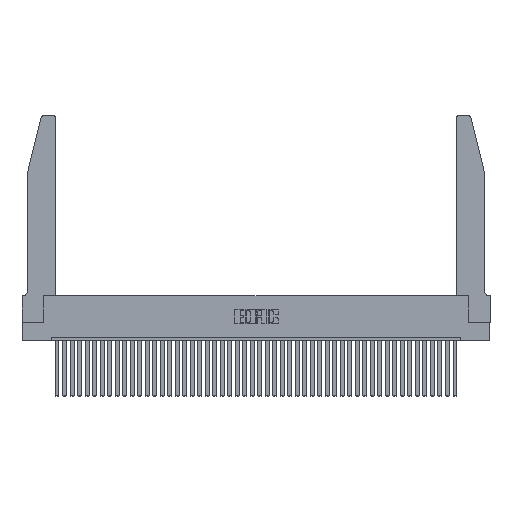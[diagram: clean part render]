
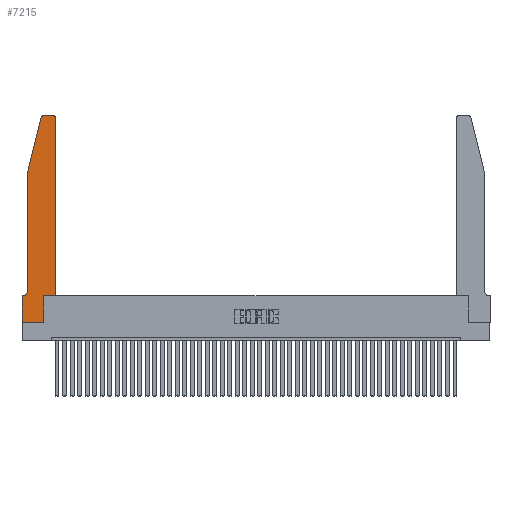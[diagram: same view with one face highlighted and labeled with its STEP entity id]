
A CAD part, top view. The second image highlights one B-rep face of the part: STEP entity #7215.
In plain terms, the highlighted planar face has unit normal (0, 0, 1).
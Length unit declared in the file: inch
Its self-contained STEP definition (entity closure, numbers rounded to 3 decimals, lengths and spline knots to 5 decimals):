
#694 = EDGE_CURVE ( 'NONE', #32693, #29416, #7862, .T. ) ;
#701 = ORIENTED_EDGE ( 'NONE', *, *, #22088, .T. ) ;
#1404 = ORIENTED_EDGE ( 'NONE', *, *, #17698, .T. ) ;
#2934 = DIRECTION ( 'NONE',  ( 0., 1., 0. ) ) ;
#3027 = LINE ( 'NONE', #38207, #21417 ) ;
#3034 = LINE ( 'NONE', #43429, #11367 ) ;
#3862 = CARTESIAN_POINT ( 'NONE',  ( 0., 0.35, 0.37 ) ) ;
#4393 = DIRECTION ( 'NONE',  ( 0., -1., 0. ) ) ;
#4620 = VERTEX_POINT ( 'NONE', #35564 ) ;
#6170 = AXIS2_PLACEMENT_3D ( 'NONE', #19109, #12069, #29299 ) ;
#6449 = DIRECTION ( 'NONE',  ( 1., 0., 0. ) ) ;
#6602 = DIRECTION ( 'NONE',  ( -1., 0., 0. ) ) ;
#6621 = CARTESIAN_POINT ( 'NONE',  ( 0.0755, 2., 0.37 ) ) ;
#7215 = ADVANCED_FACE ( 'NONE', ( #33334 ), #41296, .T. ) ;
#7603 = CARTESIAN_POINT ( 'NONE',  ( 0.4505, 0.35, 0.37 ) ) ;
#7617 = EDGE_CURVE ( 'NONE', #22363, #28635, #35387, .T. ) ;
#7655 = CARTESIAN_POINT ( 'NONE',  ( 0.0055, 0.35, 0.37 ) ) ;
#7862 = LINE ( 'NONE', #22593, #30487 ) ;
#8465 = CIRCLE ( 'NONE', #6170, 0.03 ) ;
#8792 = EDGE_CURVE ( 'NONE', #29025, #22363, #8465, .T. ) ;
#9102 = DIRECTION ( 'NONE',  ( -1., 0., 0. ) ) ;
#10351 = DIRECTION ( 'NONE',  ( -1., 0., 0. ) ) ;
#10827 = CARTESIAN_POINT ( 'NONE',  ( 0.4205, 2.75, 0.37 ) ) ;
#11204 = DIRECTION ( 'NONE',  ( 0., -1., 0. ) ) ;
#11269 = EDGE_CURVE ( 'NONE', #28635, #43336, #35503, .T. ) ;
#11367 = VECTOR ( 'NONE', #23427, 39.37008 ) ;
#12069 = DIRECTION ( 'NONE',  ( 0., 0., 1. ) ) ;
#12207 = ORIENTED_EDGE ( 'NONE', *, *, #25436, .T. ) ;
#12264 = ORIENTED_EDGE ( 'NONE', *, *, #694, .T. ) ;
#14190 = DIRECTION ( 'NONE',  ( -0.239, -0.971, 0. ) ) ;
#15334 = VECTOR ( 'NONE', #6602, 39.37008 ) ;
#15823 = CIRCLE ( 'NONE', #33012, 0.07 ) ;
#15952 = VECTOR ( 'NONE', #14190, 39.37008 ) ;
#16179 = LINE ( 'NONE', #31342, #36717 ) ;
#17528 = LINE ( 'NONE', #6621, #15952 ) ;
#17698 = EDGE_CURVE ( 'NONE', #43336, #4620, #17528, .T. ) ;
#17718 = DIRECTION ( 'NONE',  ( 0., 1., 0. ) ) ;
#19077 = CARTESIAN_POINT ( 'NONE',  ( 0.0055, 0.42, 0.37 ) ) ;
#19109 = CARTESIAN_POINT ( 'NONE',  ( 0.4205, 2.72, 0.37 ) ) ;
#19134 = CARTESIAN_POINT ( 'NONE',  ( 0., 0., 0.37 ) ) ;
#19606 = CARTESIAN_POINT ( 'NONE',  ( 0.0755, 0.42, 0.37 ) ) ;
#20384 = CARTESIAN_POINT ( 'NONE',  ( 0.0755, 0.35, 0.37 ) ) ;
#20765 = EDGE_CURVE ( 'NONE', #24609, #32693, #16179, .T. ) ;
#20997 = CARTESIAN_POINT ( 'NONE',  ( 0.25487, 2.72718, 0.37 ) ) ;
#21012 = CARTESIAN_POINT ( 'NONE',  ( 0., 0.35, 0.37 ) ) ;
#21417 = VECTOR ( 'NONE', #4393, 39.37008 ) ;
#21872 = LINE ( 'NONE', #7603, #32920 ) ;
#22088 = EDGE_CURVE ( 'NONE', #29416, #31318, #23519, .T. ) ;
#22324 = ORIENTED_EDGE ( 'NONE', *, *, #22340, .T. ) ;
#22340 = EDGE_CURVE ( 'NONE', #31322, #29025, #21872, .T. ) ;
#22363 = VERTEX_POINT ( 'NONE', #10827 ) ;
#22593 = CARTESIAN_POINT ( 'NONE',  ( 0., 0., 0.37 ) ) ;
#22949 = EDGE_CURVE ( 'NONE', #35467, #24609, #33315, .T. ) ;
#23017 = EDGE_CURVE ( 'NONE', #31318, #31322, #3034, .T. ) ;
#23427 = DIRECTION ( 'NONE',  ( 1., 0., 0. ) ) ;
#23519 = LINE ( 'NONE', #35558, #30806 ) ;
#23872 = CARTESIAN_POINT ( 'NONE',  ( 0.4505, 2.72, 0.37 ) ) ;
#24609 = VERTEX_POINT ( 'NONE', #3862 ) ;
#24851 = ORIENTED_EDGE ( 'NONE', *, *, #22949, .T. ) ;
#25256 = AXIS2_PLACEMENT_3D ( 'NONE', #21012, #41873, #28077 ) ;
#25436 = EDGE_CURVE ( 'NONE', #4620, #35775, #3027, .T. ) ;
#25988 = ORIENTED_EDGE ( 'NONE', *, *, #23017, .T. ) ;
#26732 = ORIENTED_EDGE ( 'NONE', *, *, #8792, .T. ) ;
#28077 = DIRECTION ( 'NONE',  ( 1., 0., 0. ) ) ;
#28081 = ORIENTED_EDGE ( 'NONE', *, *, #7617, .T. ) ;
#28519 = EDGE_LOOP ( 'NONE', ( #28081, #43426, #1404, #12207, #28932, #24851, #30446, #12264, #701, #25988, #22324, #26732 ) ) ;
#28635 = VERTEX_POINT ( 'NONE', #40340 ) ;
#28932 = ORIENTED_EDGE ( 'NONE', *, *, #42380, .T. ) ;
#29025 = VERTEX_POINT ( 'NONE', #23872 ) ;
#29262 = DIRECTION ( 'NONE',  ( 0., 0., -1. ) ) ;
#29299 = DIRECTION ( 'NONE',  ( 1., 0., 0. ) ) ;
#29416 = VERTEX_POINT ( 'NONE', #31203 ) ;
#30047 = CARTESIAN_POINT ( 'NONE',  ( 0.2865, 0.35, 0.37 ) ) ;
#30360 = CARTESIAN_POINT ( 'NONE',  ( 0.2605, 2.75, 0.37 ) ) ;
#30446 = ORIENTED_EDGE ( 'NONE', *, *, #20765, .T. ) ;
#30487 = VECTOR ( 'NONE', #33317, 39.37008 ) ;
#30806 = VECTOR ( 'NONE', #2934, 39.37008 ) ;
#31203 = CARTESIAN_POINT ( 'NONE',  ( 0.2865, 0., 0.37 ) ) ;
#31318 = VERTEX_POINT ( 'NONE', #30047 ) ;
#31322 = VERTEX_POINT ( 'NONE', #33692 ) ;
#31342 = CARTESIAN_POINT ( 'NONE',  ( 0., 0., 0.37 ) ) ;
#32112 = DIRECTION ( 'NONE',  ( 0., 0., 1. ) ) ;
#32693 = VERTEX_POINT ( 'NONE', #19134 ) ;
#32920 = VECTOR ( 'NONE', #17718, 39.37008 ) ;
#33012 = AXIS2_PLACEMENT_3D ( 'NONE', #19077, #29262, #9102 ) ;
#33315 = LINE ( 'NONE', #20384, #15334 ) ;
#33317 = DIRECTION ( 'NONE',  ( 1., 0., 0. ) ) ;
#33334 = FACE_OUTER_BOUND ( 'NONE', #28519, .T. ) ;
#33692 = CARTESIAN_POINT ( 'NONE',  ( 0.4505, 0.35, 0.37 ) ) ;
#35387 = LINE ( 'NONE', #30360, #43320 ) ;
#35467 = VERTEX_POINT ( 'NONE', #7655 ) ;
#35503 = CIRCLE ( 'NONE', #42525, 0.03 ) ;
#35558 = CARTESIAN_POINT ( 'NONE',  ( 0.2865, 0.35, 0.37 ) ) ;
#35564 = CARTESIAN_POINT ( 'NONE',  ( 0.0755, 2., 0.37 ) ) ;
#35775 = VERTEX_POINT ( 'NONE', #19606 ) ;
#36717 = VECTOR ( 'NONE', #11204, 39.37008 ) ;
#38207 = CARTESIAN_POINT ( 'NONE',  ( 0.0755, 2., 0.37 ) ) ;
#40340 = CARTESIAN_POINT ( 'NONE',  ( 0.284, 2.75, 0.37 ) ) ;
#41296 = PLANE ( 'NONE',  #25256 ) ;
#41873 = DIRECTION ( 'NONE',  ( 0., 0., 1. ) ) ;
#42380 = EDGE_CURVE ( 'NONE', #35775, #35467, #15823, .T. ) ;
#42525 = AXIS2_PLACEMENT_3D ( 'NONE', #43240, #32112, #6449 ) ;
#43240 = CARTESIAN_POINT ( 'NONE',  ( 0.284, 2.72, 0.37 ) ) ;
#43320 = VECTOR ( 'NONE', #10351, 39.37008 ) ;
#43336 = VERTEX_POINT ( 'NONE', #20997 ) ;
#43426 = ORIENTED_EDGE ( 'NONE', *, *, #11269, .T. ) ;
#43429 = CARTESIAN_POINT ( 'NONE',  ( 0.4505, 0.35, 0.37 ) ) ;
